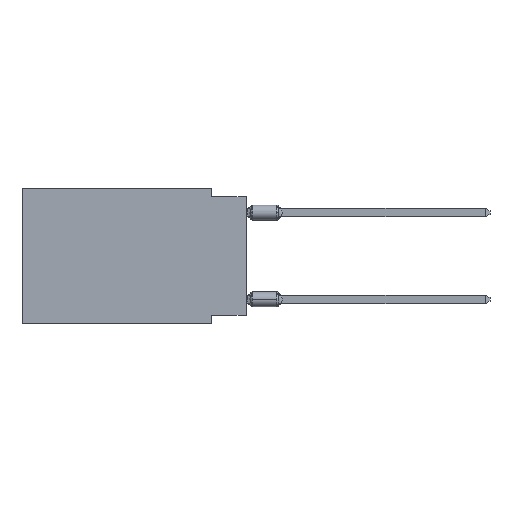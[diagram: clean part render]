
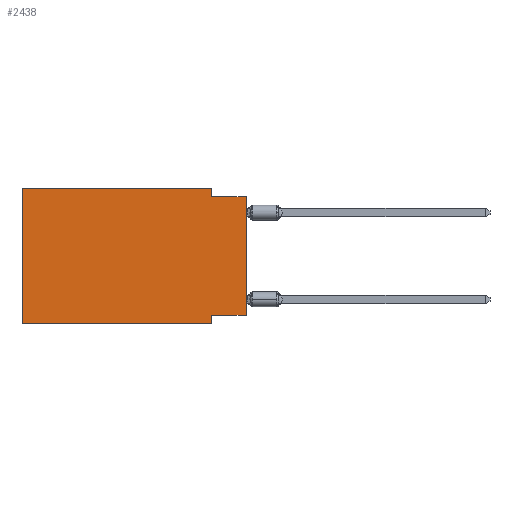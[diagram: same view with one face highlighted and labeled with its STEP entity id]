
A CAD part, left-side view. The second image highlights one B-rep face of the part: STEP entity #2438.
In plain terms, the highlighted planar face has unit normal (-1, 0, 0).
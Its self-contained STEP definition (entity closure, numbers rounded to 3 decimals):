
#452 = DIRECTION ( 'NONE',  ( 0., 0., -1. ) ) ;
#503 = ORIENTED_EDGE ( 'NONE', *, *, #4069, .T. ) ;
#785 = PLANE ( 'NONE',  #9092 ) ;
#892 = ORIENTED_EDGE ( 'NONE', *, *, #12688, .F. ) ;
#997 = CARTESIAN_POINT ( 'NONE',  ( 0., 16.383, 0. ) ) ;
#1240 = VECTOR ( 'NONE', #3972, 1000. ) ;
#1359 = VERTEX_POINT ( 'NONE', #10396 ) ;
#1398 = VERTEX_POINT ( 'NONE', #6341 ) ;
#1447 = CARTESIAN_POINT ( 'NONE',  ( 0., 2.54, -9.271 ) ) ;
#1787 = CARTESIAN_POINT ( 'NONE',  ( 0., 0., -9.271 ) ) ;
#2226 = CARTESIAN_POINT ( 'NONE',  ( 0., 2.54, 0. ) ) ;
#2438 = ADVANCED_FACE ( 'NONE', ( #11723 ), #785, .F. ) ;
#2483 = CARTESIAN_POINT ( 'NONE',  ( 0., 0., -0.635 ) ) ;
#2543 = EDGE_CURVE ( 'NONE', #1359, #7649, #8319, .T. ) ;
#2583 = CARTESIAN_POINT ( 'NONE',  ( 0., 16.383, 0. ) ) ;
#2799 = ORIENTED_EDGE ( 'NONE', *, *, #7656, .F. ) ;
#3006 = CARTESIAN_POINT ( 'NONE',  ( 0., 16.383, 0. ) ) ;
#3141 = VERTEX_POINT ( 'NONE', #997 ) ;
#3454 = ORIENTED_EDGE ( 'NONE', *, *, #9676, .F. ) ;
#3755 = ORIENTED_EDGE ( 'NONE', *, *, #10634, .T. ) ;
#3774 = DIRECTION ( 'NONE',  ( 0., 1., 0. ) ) ;
#3802 = CARTESIAN_POINT ( 'NONE',  ( 0., 16.383, -9.906 ) ) ;
#3972 = DIRECTION ( 'NONE',  ( 0., 0., 1. ) ) ;
#4069 = EDGE_CURVE ( 'NONE', #7319, #8749, #9539, .T. ) ;
#4823 = LINE ( 'NONE', #2583, #11986 ) ;
#5261 = VECTOR ( 'NONE', #7729, 1000. ) ;
#5671 = CARTESIAN_POINT ( 'NONE',  ( 0., 16.383, -9.906 ) ) ;
#6248 = VERTEX_POINT ( 'NONE', #1787 ) ;
#6341 = CARTESIAN_POINT ( 'NONE',  ( 0., 0., -0.635 ) ) ;
#6568 = VERTEX_POINT ( 'NONE', #1447 ) ;
#6790 = VECTOR ( 'NONE', #7334, 1000. ) ;
#6812 = CARTESIAN_POINT ( 'NONE',  ( 0., 0., -9.271 ) ) ;
#7275 = VECTOR ( 'NONE', #3774, 1000. ) ;
#7319 = VERTEX_POINT ( 'NONE', #3802 ) ;
#7334 = DIRECTION ( 'NONE',  ( 0., 0., -1. ) ) ;
#7531 = LINE ( 'NONE', #2483, #10433 ) ;
#7631 = DIRECTION ( 'NONE',  ( 0., -1., 0. ) ) ;
#7634 = ORIENTED_EDGE ( 'NONE', *, *, #11602, .F. ) ;
#7649 = VERTEX_POINT ( 'NONE', #9629 ) ;
#7656 = EDGE_CURVE ( 'NONE', #3141, #1359, #12911, .T. ) ;
#7729 = DIRECTION ( 'NONE',  ( 0., -1., 0. ) ) ;
#7907 = EDGE_CURVE ( 'NONE', #6568, #8749, #8443, .T. ) ;
#8319 = LINE ( 'NONE', #2226, #6790 ) ;
#8443 = LINE ( 'NONE', #11273, #11113 ) ;
#8609 = DIRECTION ( 'NONE',  ( 0., 0., 1. ) ) ;
#8634 = ORIENTED_EDGE ( 'NONE', *, *, #7907, .F. ) ;
#8749 = VERTEX_POINT ( 'NONE', #10614 ) ;
#8962 = LINE ( 'NONE', #12115, #1240 ) ;
#8963 = LINE ( 'NONE', #6812, #7275 ) ;
#9092 = AXIS2_PLACEMENT_3D ( 'NONE', #3006, #12775, #10879 ) ;
#9539 = LINE ( 'NONE', #5671, #9706 ) ;
#9629 = CARTESIAN_POINT ( 'NONE',  ( 0., 2.54, -0.635 ) ) ;
#9676 = EDGE_CURVE ( 'NONE', #7319, #3141, #4823, .T. ) ;
#9706 = VECTOR ( 'NONE', #7631, 1000. ) ;
#10396 = CARTESIAN_POINT ( 'NONE',  ( 0., 2.54, 0. ) ) ;
#10433 = VECTOR ( 'NONE', #10603, 1000. ) ;
#10603 = DIRECTION ( 'NONE',  ( 0., -1., 0. ) ) ;
#10614 = CARTESIAN_POINT ( 'NONE',  ( 0., 2.54, -9.906 ) ) ;
#10634 = EDGE_CURVE ( 'NONE', #6248, #1398, #8962, .T. ) ;
#10668 = ORIENTED_EDGE ( 'NONE', *, *, #2543, .F. ) ;
#10879 = DIRECTION ( 'NONE',  ( 0., 0., -1. ) ) ;
#11113 = VECTOR ( 'NONE', #452, 1000. ) ;
#11273 = CARTESIAN_POINT ( 'NONE',  ( 0., 2.54, -9.906 ) ) ;
#11602 = EDGE_CURVE ( 'NONE', #6248, #6568, #8963, .T. ) ;
#11723 = FACE_OUTER_BOUND ( 'NONE', #11934, .T. ) ;
#11934 = EDGE_LOOP ( 'NONE', ( #3755, #892, #10668, #2799, #3454, #503, #8634, #7634 ) ) ;
#11986 = VECTOR ( 'NONE', #8609, 1000. ) ;
#12115 = CARTESIAN_POINT ( 'NONE',  ( 0., 0., 0. ) ) ;
#12643 = CARTESIAN_POINT ( 'NONE',  ( 0., 16.383, 0. ) ) ;
#12688 = EDGE_CURVE ( 'NONE', #7649, #1398, #7531, .T. ) ;
#12775 = DIRECTION ( 'NONE',  ( 1., 0., 0. ) ) ;
#12911 = LINE ( 'NONE', #12643, #5261 ) ;
